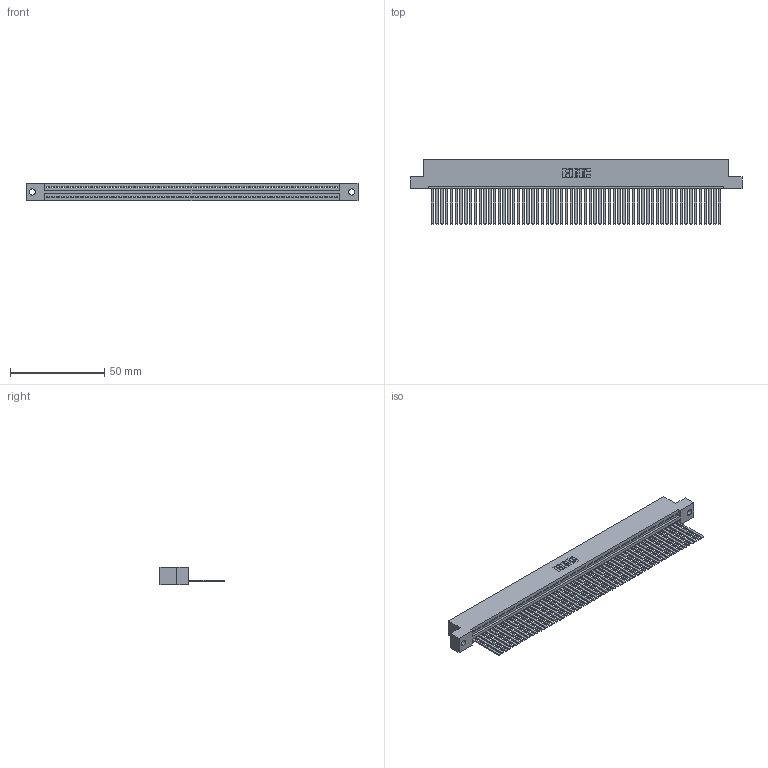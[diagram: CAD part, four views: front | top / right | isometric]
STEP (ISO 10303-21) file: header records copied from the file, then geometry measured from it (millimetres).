
FILE_DESCRIPTION (( 'STEP AP203' ), '1' );
FILE_NAME ('395-061-544-102.STEP', '2019-10-24T15:57:09', ( '' ), ( '' ), 'SwSTEP 2.0', 'SolidWorks 2016', '' );
FILE_SCHEMA (( 'CONFIG_CONTROL_DESIGN' ));
Length unit declared in the file: inch
Products named in the file (3): 395-061-544-102; 345-292-001_345-293-144; 345 Part_Flush Mounting Lugs - 0.128 Dia
Assembly tree (62 placements, depth 2):
  395-061-544-102
    345 Part_Flush Mounting Lugs - 0.128 Dia
    345-292-001_345-293-144  x61
Bounding box: 176.15 x 33.96 x 9.4 mm (x, y, z)
Volume: 17556.2 mm3; surface area: 25438.2 mm2
Topology: 62 solids, 62 shells, 3298 faces, 9979 edges, 6570 vertices
Faces by surface type: plane 2276, cylinder 1022
Entity records: 43171 total; most frequent: CARTESIAN_POINT 7483, ORIENTED_EDGE 7478, DIRECTION 6505, EDGE_CURVE 3739, LINE 3367, VECTOR 3367, VERTEX_POINT 2490, AXIS2_PLACEMENT_3D 1569
